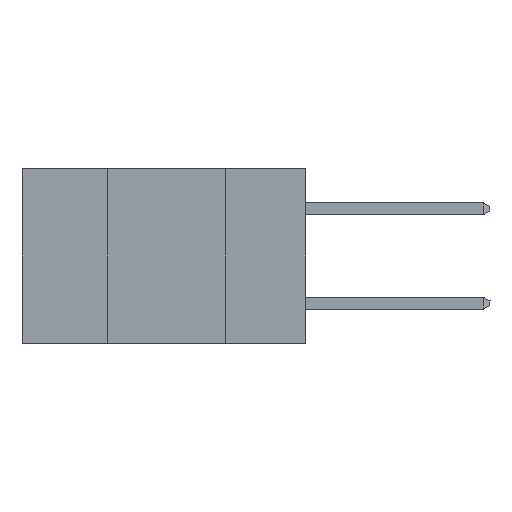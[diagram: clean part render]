
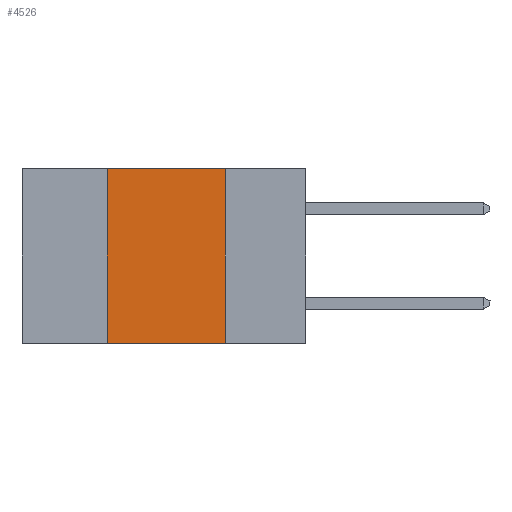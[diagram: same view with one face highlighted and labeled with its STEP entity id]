
A CAD part, left-side view. The second image highlights one B-rep face of the part: STEP entity #4526.
In plain terms, the highlighted planar face has unit normal (-1, 0, 0).
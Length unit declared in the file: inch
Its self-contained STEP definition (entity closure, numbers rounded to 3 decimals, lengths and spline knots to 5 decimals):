
#558 = CARTESIAN_POINT ( 'NONE',  ( 0., 0.6, 0. ) ) ;
#628 = ORIENTED_EDGE ( 'NONE', *, *, #18346, .T. ) ;
#3042 = LINE ( 'NONE', #16104, #9674 ) ;
#3254 = VERTEX_POINT ( 'NONE', #24248 ) ;
#3748 = VECTOR ( 'NONE', #23601, 39.37008 ) ;
#4526 = ADVANCED_FACE ( 'NONE', ( #15395 ), #20180, .F. ) ;
#6966 = VERTEX_POINT ( 'NONE', #8567 ) ;
#7734 = EDGE_CURVE ( 'NONE', #3254, #19804, #25463, .T. ) ;
#8567 = CARTESIAN_POINT ( 'NONE',  ( 0., 0.17, -0.37 ) ) ;
#9674 = VECTOR ( 'NONE', #16530, 39.37008 ) ;
#9882 = DIRECTION ( 'NONE',  ( 0., 0., -1. ) ) ;
#11832 = CARTESIAN_POINT ( 'NONE',  ( 0., 0.6, 0. ) ) ;
#12133 = EDGE_CURVE ( 'NONE', #13704, #6966, #23996, .T. ) ;
#13403 = DIRECTION ( 'NONE',  ( 0., 0., 1. ) ) ;
#13704 = VERTEX_POINT ( 'NONE', #24045 ) ;
#14152 = ORIENTED_EDGE ( 'NONE', *, *, #19693, .F. ) ;
#15294 = AXIS2_PLACEMENT_3D ( 'NONE', #11832, #24298, #9882 ) ;
#15395 = FACE_OUTER_BOUND ( 'NONE', #15850, .T. ) ;
#15850 = EDGE_LOOP ( 'NONE', ( #22295, #14152, #26271, #628 ) ) ;
#16104 = CARTESIAN_POINT ( 'NONE',  ( 0., 0.6, -0.37 ) ) ;
#16530 = DIRECTION ( 'NONE',  ( 0., -1., 0. ) ) ;
#17438 = CARTESIAN_POINT ( 'NONE',  ( 0., 0.17, 0. ) ) ;
#18216 = VECTOR ( 'NONE', #24849, 39.37008 ) ;
#18346 = EDGE_CURVE ( 'NONE', #3254, #6966, #3042, .T. ) ;
#18705 = LINE ( 'NONE', #558, #18216 ) ;
#18854 = VECTOR ( 'NONE', #13403, 39.37008 ) ;
#19693 = EDGE_CURVE ( 'NONE', #19804, #13704, #18705, .T. ) ;
#19804 = VERTEX_POINT ( 'NONE', #24437 ) ;
#20180 = PLANE ( 'NONE',  #15294 ) ;
#21367 = CARTESIAN_POINT ( 'NONE',  ( 0., 0.42, 0. ) ) ;
#22295 = ORIENTED_EDGE ( 'NONE', *, *, #12133, .F. ) ;
#23601 = DIRECTION ( 'NONE',  ( 0., 0., -1. ) ) ;
#23996 = LINE ( 'NONE', #17438, #3748 ) ;
#24045 = CARTESIAN_POINT ( 'NONE',  ( 0., 0.17, 0. ) ) ;
#24248 = CARTESIAN_POINT ( 'NONE',  ( 0., 0.42, -0.37 ) ) ;
#24298 = DIRECTION ( 'NONE',  ( 1., 0., 0. ) ) ;
#24437 = CARTESIAN_POINT ( 'NONE',  ( 0., 0.42, 0. ) ) ;
#24849 = DIRECTION ( 'NONE',  ( 0., -1., 0. ) ) ;
#25463 = LINE ( 'NONE', #21367, #18854 ) ;
#26271 = ORIENTED_EDGE ( 'NONE', *, *, #7734, .F. ) ;
